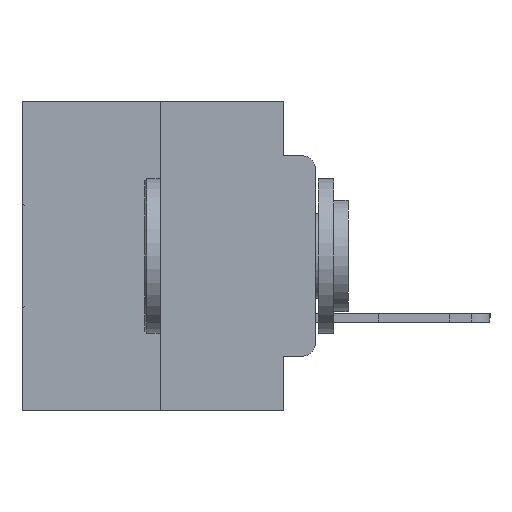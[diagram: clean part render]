
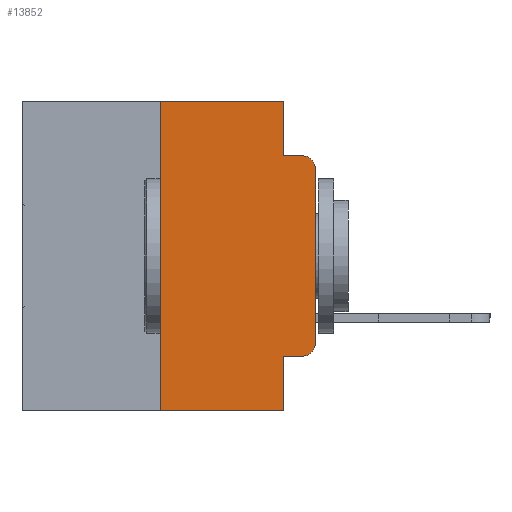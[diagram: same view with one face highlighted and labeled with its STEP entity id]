
A CAD part, left-side view. The second image highlights one B-rep face of the part: STEP entity #13852.
In plain terms, the highlighted planar face has unit normal (-1, 0, 0).
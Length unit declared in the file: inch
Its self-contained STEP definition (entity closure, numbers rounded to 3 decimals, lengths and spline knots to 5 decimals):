
#257 = LINE ( 'NONE', #14578, #6668 ) ;
#326 = DIRECTION ( 'NONE',  ( -1., 0., 0. ) ) ;
#573 = VERTEX_POINT ( 'NONE', #25190 ) ;
#1612 = VERTEX_POINT ( 'NONE', #10705 ) ;
#2114 = VECTOR ( 'NONE', #18562, 39.37008 ) ;
#2639 = DIRECTION ( 'NONE',  ( -1., 0., 0. ) ) ;
#3229 = EDGE_LOOP ( 'NONE', ( #24809, #14982, #13545, #26858, #24492, #27252, #10670, #5969, #26540, #18226 ) ) ;
#3473 = LINE ( 'NONE', #24616, #15877 ) ;
#3877 = CARTESIAN_POINT ( 'NONE',  ( 0., 0.473, 0. ) ) ;
#4626 = CARTESIAN_POINT ( 'NONE',  ( 0., 0.25, -0.5 ) ) ;
#4791 = CARTESIAN_POINT ( 'NONE',  ( 0., 0.02, -0.0885 ) ) ;
#5384 = CARTESIAN_POINT ( 'NONE',  ( 0., 0.473, 0. ) ) ;
#5471 = CARTESIAN_POINT ( 'NONE',  ( 0., 0.051, 0. ) ) ;
#5969 = ORIENTED_EDGE ( 'NONE', *, *, #10290, .F. ) ;
#6274 = DIRECTION ( 'NONE',  ( 0., -1., 0. ) ) ;
#6362 = VERTEX_POINT ( 'NONE', #19943 ) ;
#6562 = DIRECTION ( 'NONE',  ( 0., -1., 0. ) ) ;
#6668 = VECTOR ( 'NONE', #9991, 39.37008 ) ;
#6896 = CARTESIAN_POINT ( 'NONE',  ( 0., 0.473, -0.5 ) ) ;
#7180 = LINE ( 'NONE', #3877, #24563 ) ;
#7185 = EDGE_CURVE ( 'NONE', #1612, #6362, #12667, .T. ) ;
#7295 = VERTEX_POINT ( 'NONE', #27900 ) ;
#7625 = CARTESIAN_POINT ( 'NONE',  ( 0., 0.051, -0.4115 ) ) ;
#7716 = VERTEX_POINT ( 'NONE', #4791 ) ;
#7741 = DIRECTION ( 'NONE',  ( 1., 0., 0. ) ) ;
#7893 = AXIS2_PLACEMENT_3D ( 'NONE', #16630, #2639, #18886 ) ;
#8518 = VERTEX_POINT ( 'NONE', #17898 ) ;
#8649 = VERTEX_POINT ( 'NONE', #4626 ) ;
#8771 = EDGE_CURVE ( 'NONE', #8518, #1612, #13672, .T. ) ;
#8990 = EDGE_CURVE ( 'NONE', #11687, #16882, #7180, .T. ) ;
#9978 = DIRECTION ( 'NONE',  ( 0., -1., 0. ) ) ;
#9991 = DIRECTION ( 'NONE',  ( 0., 0., 1. ) ) ;
#10290 = EDGE_CURVE ( 'NONE', #8518, #28985, #28833, .T. ) ;
#10670 = ORIENTED_EDGE ( 'NONE', *, *, #10675, .T. ) ;
#10675 = EDGE_CURVE ( 'NONE', #8649, #28985, #19982, .T. ) ;
#10705 = CARTESIAN_POINT ( 'NONE',  ( 0., 0.02, -0.4115 ) ) ;
#11088 = VECTOR ( 'NONE', #19447, 39.37008 ) ;
#11127 = DIRECTION ( 'NONE',  ( 0., 0., 1. ) ) ;
#11273 = CARTESIAN_POINT ( 'NONE',  ( 0., 0.051, 0. ) ) ;
#11687 = VERTEX_POINT ( 'NONE', #18092 ) ;
#11839 = EDGE_CURVE ( 'NONE', #8649, #11687, #257, .T. ) ;
#12667 = CIRCLE ( 'NONE', #7893, 0.02 ) ;
#13355 = VECTOR ( 'NONE', #6562, 39.37008 ) ;
#13545 = ORIENTED_EDGE ( 'NONE', *, *, #17981, .F. ) ;
#13672 = LINE ( 'NONE', #7625, #25611 ) ;
#13852 = ADVANCED_FACE ( 'NONE', ( #24296 ), #19162, .F. ) ;
#14383 = CARTESIAN_POINT ( 'NONE',  ( 0., 0.02, -0.1085 ) ) ;
#14578 = CARTESIAN_POINT ( 'NONE',  ( 0., 0.25, 0. ) ) ;
#14982 = ORIENTED_EDGE ( 'NONE', *, *, #19478, .T. ) ;
#15720 = CARTESIAN_POINT ( 'NONE',  ( 0., 0.051, -0.0885 ) ) ;
#15877 = VECTOR ( 'NONE', #11127, 39.37008 ) ;
#16462 = EDGE_CURVE ( 'NONE', #16882, #573, #20586, .T. ) ;
#16630 = CARTESIAN_POINT ( 'NONE',  ( 0., 0.02, -0.3915 ) ) ;
#16724 = DIRECTION ( 'NONE',  ( 0., 0., -1. ) ) ;
#16882 = VERTEX_POINT ( 'NONE', #18488 ) ;
#17266 = CIRCLE ( 'NONE', #25867, 0.02 ) ;
#17898 = CARTESIAN_POINT ( 'NONE',  ( 0., 0.051, -0.4115 ) ) ;
#17981 = EDGE_CURVE ( 'NONE', #573, #7716, #19443, .T. ) ;
#18092 = CARTESIAN_POINT ( 'NONE',  ( 0., 0.25, 0. ) ) ;
#18226 = ORIENTED_EDGE ( 'NONE', *, *, #7185, .T. ) ;
#18488 = CARTESIAN_POINT ( 'NONE',  ( 0., 0.051, 0. ) ) ;
#18562 = DIRECTION ( 'NONE',  ( 0., 0., -1. ) ) ;
#18886 = DIRECTION ( 'NONE',  ( 0., 0., -1. ) ) ;
#19162 = PLANE ( 'NONE',  #21127 ) ;
#19274 = VECTOR ( 'NONE', #25028, 39.37008 ) ;
#19443 = LINE ( 'NONE', #15720, #13355 ) ;
#19447 = DIRECTION ( 'NONE',  ( 0., 0., -1. ) ) ;
#19478 = EDGE_CURVE ( 'NONE', #7295, #7716, #17266, .T. ) ;
#19943 = CARTESIAN_POINT ( 'NONE',  ( 0., 0., -0.3915 ) ) ;
#19982 = LINE ( 'NONE', #6896, #19274 ) ;
#20586 = LINE ( 'NONE', #11273, #2114 ) ;
#20959 = EDGE_CURVE ( 'NONE', #6362, #7295, #3473, .T. ) ;
#21127 = AXIS2_PLACEMENT_3D ( 'NONE', #5384, #7741, #23608 ) ;
#23608 = DIRECTION ( 'NONE',  ( 0., 0., -1. ) ) ;
#24296 = FACE_OUTER_BOUND ( 'NONE', #3229, .T. ) ;
#24492 = ORIENTED_EDGE ( 'NONE', *, *, #8990, .F. ) ;
#24563 = VECTOR ( 'NONE', #6274, 39.37008 ) ;
#24616 = CARTESIAN_POINT ( 'NONE',  ( 0., 0., 0. ) ) ;
#24809 = ORIENTED_EDGE ( 'NONE', *, *, #20959, .T. ) ;
#25028 = DIRECTION ( 'NONE',  ( 0., -1., 0. ) ) ;
#25190 = CARTESIAN_POINT ( 'NONE',  ( 0., 0.051, -0.0885 ) ) ;
#25611 = VECTOR ( 'NONE', #9978, 39.37008 ) ;
#25867 = AXIS2_PLACEMENT_3D ( 'NONE', #14383, #326, #16724 ) ;
#26540 = ORIENTED_EDGE ( 'NONE', *, *, #8771, .T. ) ;
#26858 = ORIENTED_EDGE ( 'NONE', *, *, #16462, .F. ) ;
#27252 = ORIENTED_EDGE ( 'NONE', *, *, #11839, .F. ) ;
#27900 = CARTESIAN_POINT ( 'NONE',  ( 0., 0., -0.1085 ) ) ;
#28343 = CARTESIAN_POINT ( 'NONE',  ( 0., 0.051, -0.5 ) ) ;
#28833 = LINE ( 'NONE', #5471, #11088 ) ;
#28985 = VERTEX_POINT ( 'NONE', #28343 ) ;
